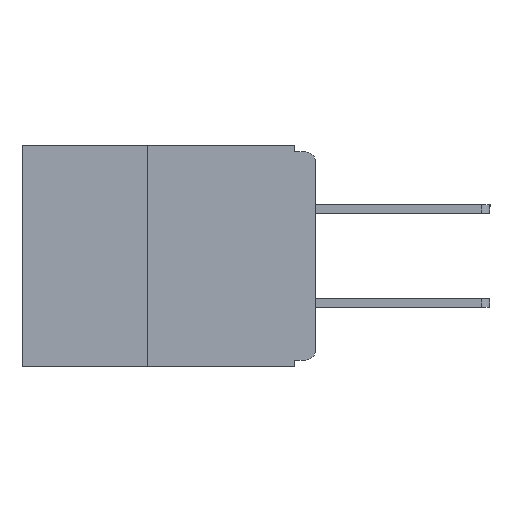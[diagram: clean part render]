
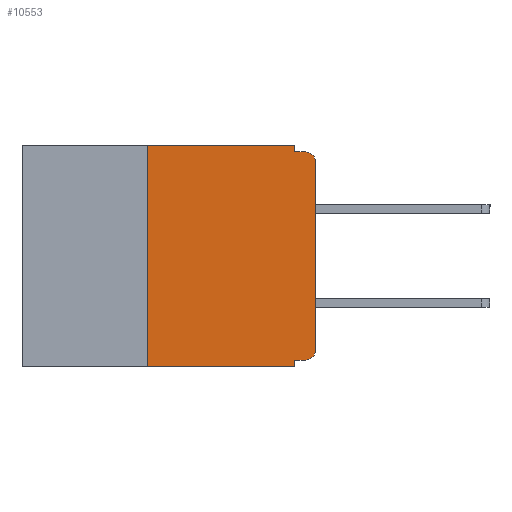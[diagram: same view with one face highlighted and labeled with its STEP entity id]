
A CAD part, left-side view. The second image highlights one B-rep face of the part: STEP entity #10553.
In plain terms, the highlighted planar face has unit normal (-1, 0, 0).
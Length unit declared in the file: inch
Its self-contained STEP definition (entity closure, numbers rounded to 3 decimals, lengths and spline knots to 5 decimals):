
#50 = CARTESIAN_POINT ( 'NONE',  ( 0., 0., 0. ) ) ;
#358 = ORIENTED_EDGE ( 'NONE', *, *, #1525, .F. ) ;
#366 = DIRECTION ( 'NONE',  ( 0., -1., 0. ) ) ;
#471 = VECTOR ( 'NONE', #1606, 39.37008 ) ;
#849 = LINE ( 'NONE', #14568, #471 ) ;
#869 = DIRECTION ( 'NONE',  ( 0., 0., 1. ) ) ;
#870 = DIRECTION ( 'NONE',  ( 0., 0., -1. ) ) ;
#876 = DIRECTION ( 'NONE',  ( 0., 0., -1. ) ) ;
#1164 = VERTEX_POINT ( 'NONE', #11281 ) ;
#1178 = ORIENTED_EDGE ( 'NONE', *, *, #2893, .T. ) ;
#1525 = EDGE_CURVE ( 'NONE', #15062, #1164, #2824, .T. ) ;
#1606 = DIRECTION ( 'NONE',  ( 0., 0., -1. ) ) ;
#1810 = DIRECTION ( 'NONE',  ( 0., -1., 0. ) ) ;
#1811 = LINE ( 'NONE', #3016, #8190 ) ;
#2069 = CIRCLE ( 'NONE', #8275, 0.015 ) ;
#2315 = FACE_OUTER_BOUND ( 'NONE', #2545, .T. ) ;
#2545 = EDGE_LOOP ( 'NONE', ( #4632, #13402, #4119, #2946, #8077, #11069, #1178, #9413, #358, #12266 ) ) ;
#2824 = LINE ( 'NONE', #4336, #14940 ) ;
#2846 = LINE ( 'NONE', #13897, #6059 ) ;
#2893 = EDGE_CURVE ( 'NONE', #7837, #3620, #12095, .T. ) ;
#2946 = ORIENTED_EDGE ( 'NONE', *, *, #9770, .F. ) ;
#2993 = AXIS2_PLACEMENT_3D ( 'NONE', #3593, #11910, #4829 ) ;
#3016 = CARTESIAN_POINT ( 'NONE',  ( 0., 0.437, 0. ) ) ;
#3086 = CARTESIAN_POINT ( 'NONE',  ( 0., 0., -0.305 ) ) ;
#3187 = CARTESIAN_POINT ( 'NONE',  ( 0., 0.031, -0.01 ) ) ;
#3593 = CARTESIAN_POINT ( 'NONE',  ( 0., 0.015, -0.025 ) ) ;
#3620 = VERTEX_POINT ( 'NONE', #10122 ) ;
#3659 = VERTEX_POINT ( 'NONE', #10087 ) ;
#3754 = VERTEX_POINT ( 'NONE', #10942 ) ;
#4119 = ORIENTED_EDGE ( 'NONE', *, *, #13095, .F. ) ;
#4213 = VERTEX_POINT ( 'NONE', #3187 ) ;
#4336 = CARTESIAN_POINT ( 'NONE',  ( 0., 0., -0.32 ) ) ;
#4632 = ORIENTED_EDGE ( 'NONE', *, *, #13460, .T. ) ;
#4697 = VECTOR ( 'NONE', #869, 39.37008 ) ;
#4829 = DIRECTION ( 'NONE',  ( 0., 0., -1. ) ) ;
#5164 = VERTEX_POINT ( 'NONE', #3086 ) ;
#5415 = CARTESIAN_POINT ( 'NONE',  ( 0., 0.015, -0.305 ) ) ;
#5482 = CIRCLE ( 'NONE', #2993, 0.015 ) ;
#5721 = CARTESIAN_POINT ( 'NONE',  ( 0., 0.015, -0.32 ) ) ;
#5845 = CARTESIAN_POINT ( 'NONE',  ( 0., 0.015, -0.01 ) ) ;
#6059 = VECTOR ( 'NONE', #870, 39.37008 ) ;
#6262 = CARTESIAN_POINT ( 'NONE',  ( 0., 0.25, -0.33 ) ) ;
#6612 = DIRECTION ( 'NONE',  ( 0., 0., -1. ) ) ;
#6869 = EDGE_CURVE ( 'NONE', #1164, #3620, #2846, .T. ) ;
#6958 = CARTESIAN_POINT ( 'NONE',  ( 0., 0.25, 0. ) ) ;
#7584 = VERTEX_POINT ( 'NONE', #5845 ) ;
#7837 = VERTEX_POINT ( 'NONE', #6262 ) ;
#7850 = DIRECTION ( 'NONE',  ( 0., 1., 0. ) ) ;
#8011 = EDGE_CURVE ( 'NONE', #15062, #5164, #2069, .T. ) ;
#8030 = LINE ( 'NONE', #50, #10792 ) ;
#8077 = ORIENTED_EDGE ( 'NONE', *, *, #9915, .F. ) ;
#8099 = DIRECTION ( 'NONE',  ( 1., 0., 0. ) ) ;
#8190 = VECTOR ( 'NONE', #1810, 39.37008 ) ;
#8275 = AXIS2_PLACEMENT_3D ( 'NONE', #5415, #13628, #6612 ) ;
#9413 = ORIENTED_EDGE ( 'NONE', *, *, #6869, .F. ) ;
#9653 = DIRECTION ( 'NONE',  ( 0., 0., 1. ) ) ;
#9770 = EDGE_CURVE ( 'NONE', #3754, #4213, #849, .T. ) ;
#9915 = EDGE_CURVE ( 'NONE', #10112, #3754, #1811, .T. ) ;
#10087 = CARTESIAN_POINT ( 'NONE',  ( 0., 0., -0.025 ) ) ;
#10112 = VERTEX_POINT ( 'NONE', #6958 ) ;
#10122 = CARTESIAN_POINT ( 'NONE',  ( 0., 0.031, -0.33 ) ) ;
#10434 = VECTOR ( 'NONE', #366, 39.37008 ) ;
#10463 = CARTESIAN_POINT ( 'NONE',  ( 0., 0.25, -0.33 ) ) ;
#10553 = ADVANCED_FACE ( 'NONE', ( #2315 ), #15007, .F. ) ;
#10792 = VECTOR ( 'NONE', #9653, 39.37008 ) ;
#10942 = CARTESIAN_POINT ( 'NONE',  ( 0., 0.031, 0. ) ) ;
#11015 = LINE ( 'NONE', #10463, #4697 ) ;
#11069 = ORIENTED_EDGE ( 'NONE', *, *, #12410, .F. ) ;
#11281 = CARTESIAN_POINT ( 'NONE',  ( 0., 0.031, -0.32 ) ) ;
#11586 = CARTESIAN_POINT ( 'NONE',  ( 0., 0.437, 0. ) ) ;
#11720 = VECTOR ( 'NONE', #13356, 39.37008 ) ;
#11910 = DIRECTION ( 'NONE',  ( -1., 0., 0. ) ) ;
#11925 = EDGE_CURVE ( 'NONE', #3659, #7584, #5482, .T. ) ;
#12095 = LINE ( 'NONE', #15172, #11720 ) ;
#12266 = ORIENTED_EDGE ( 'NONE', *, *, #8011, .T. ) ;
#12410 = EDGE_CURVE ( 'NONE', #7837, #10112, #11015, .T. ) ;
#13095 = EDGE_CURVE ( 'NONE', #4213, #7584, #13526, .T. ) ;
#13356 = DIRECTION ( 'NONE',  ( 0., -1., 0. ) ) ;
#13402 = ORIENTED_EDGE ( 'NONE', *, *, #11925, .T. ) ;
#13436 = CARTESIAN_POINT ( 'NONE',  ( 0., 0., -0.01 ) ) ;
#13460 = EDGE_CURVE ( 'NONE', #5164, #3659, #8030, .T. ) ;
#13526 = LINE ( 'NONE', #13436, #10434 ) ;
#13628 = DIRECTION ( 'NONE',  ( -1., 0., 0. ) ) ;
#13897 = CARTESIAN_POINT ( 'NONE',  ( 0., 0.031, -0.33 ) ) ;
#14241 = AXIS2_PLACEMENT_3D ( 'NONE', #11586, #8099, #876 ) ;
#14568 = CARTESIAN_POINT ( 'NONE',  ( 0., 0.031, 0. ) ) ;
#14940 = VECTOR ( 'NONE', #7850, 39.37008 ) ;
#15007 = PLANE ( 'NONE',  #14241 ) ;
#15062 = VERTEX_POINT ( 'NONE', #5721 ) ;
#15172 = CARTESIAN_POINT ( 'NONE',  ( 0., 0.437, -0.33 ) ) ;
